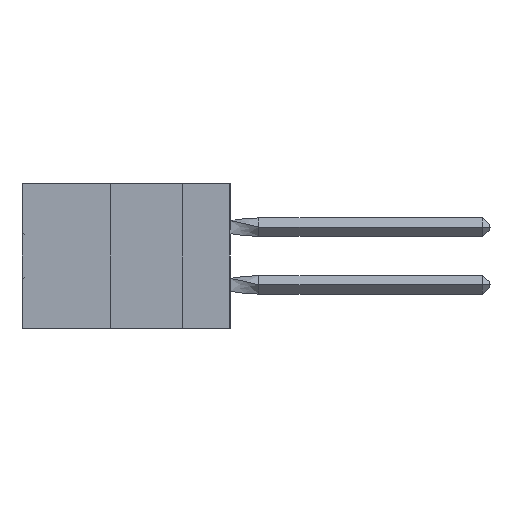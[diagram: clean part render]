
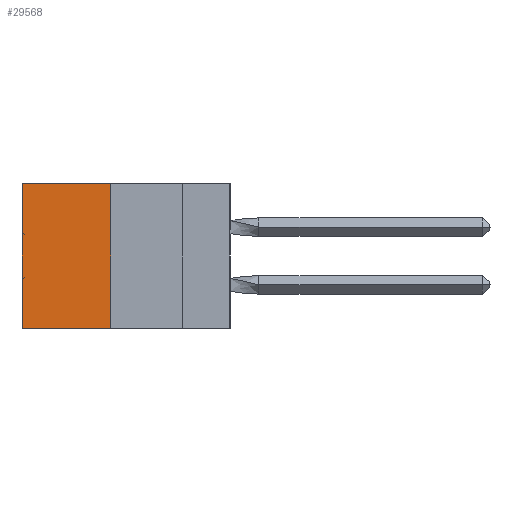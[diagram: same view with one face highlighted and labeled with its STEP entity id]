
A CAD part, left-side view. The second image highlights one B-rep face of the part: STEP entity #29568.
In plain terms, the highlighted planar face has unit normal (-1, 0, 0).
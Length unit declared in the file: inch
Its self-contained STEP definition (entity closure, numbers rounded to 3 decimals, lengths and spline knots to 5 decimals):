
#849 = VECTOR ( 'NONE', #43727, 39.37008 ) ;
#4710 = FACE_OUTER_BOUND ( 'NONE', #11921, .T. ) ;
#4960 = CARTESIAN_POINT ( 'NONE',  ( 0.305, 0.413, -0.5 ) ) ;
#6010 = ORIENTED_EDGE ( 'NONE', *, *, #20643, .F. ) ;
#6087 = EDGE_CURVE ( 'NONE', #27069, #34955, #31797, .T. ) ;
#6821 = EDGE_CURVE ( 'NONE', #34955, #45944, #55097, .T. ) ;
#7483 = ORIENTED_EDGE ( 'NONE', *, *, #6821, .T. ) ;
#8641 = VECTOR ( 'NONE', #21583, 39.37008 ) ;
#11921 = EDGE_LOOP ( 'NONE', ( #7483, #6010, #18293, #22576 ) ) ;
#12285 = PLANE ( 'NONE',  #30268 ) ;
#13831 = CARTESIAN_POINT ( 'NONE',  ( 0.305, 0.72, -0.5 ) ) ;
#15312 = DIRECTION ( 'NONE',  ( 0., 0., -1. ) ) ;
#18049 = CARTESIAN_POINT ( 'NONE',  ( 0.305, 0.72, -0.5 ) ) ;
#18293 = ORIENTED_EDGE ( 'NONE', *, *, #25201, .F. ) ;
#19469 = CARTESIAN_POINT ( 'NONE',  ( 0.305, 0.413, -0.5 ) ) ;
#19927 = CARTESIAN_POINT ( 'NONE',  ( 0.305, 0.72, 0. ) ) ;
#20467 = DIRECTION ( 'NONE',  ( 0., 1., 0. ) ) ;
#20643 = EDGE_CURVE ( 'NONE', #52674, #45944, #23427, .T. ) ;
#21583 = DIRECTION ( 'NONE',  ( 0., 1., 0. ) ) ;
#22576 = ORIENTED_EDGE ( 'NONE', *, *, #6087, .T. ) ;
#23427 = LINE ( 'NONE', #38627, #8641 ) ;
#25201 = EDGE_CURVE ( 'NONE', #27069, #52674, #27667, .T. ) ;
#27069 = VERTEX_POINT ( 'NONE', #51683 ) ;
#27148 = VECTOR ( 'NONE', #20467, 39.37008 ) ;
#27667 = LINE ( 'NONE', #19469, #48987 ) ;
#29043 = DIRECTION ( 'NONE',  ( 1., 0., 0. ) ) ;
#29229 = DIRECTION ( 'NONE',  ( 0., 0., -1. ) ) ;
#29568 = ADVANCED_FACE ( 'NONE', ( #4710 ), #12285, .F. ) ;
#30268 = AXIS2_PLACEMENT_3D ( 'NONE', #46552, #29043, #29229 ) ;
#31797 = LINE ( 'NONE', #46104, #27148 ) ;
#34955 = VERTEX_POINT ( 'NONE', #19927 ) ;
#38627 = CARTESIAN_POINT ( 'NONE',  ( 0.305, 0.413, -0.5 ) ) ;
#43727 = DIRECTION ( 'NONE',  ( 0., 0., -1. ) ) ;
#45944 = VERTEX_POINT ( 'NONE', #13831 ) ;
#46104 = CARTESIAN_POINT ( 'NONE',  ( 0.305, 0.413, 0. ) ) ;
#46552 = CARTESIAN_POINT ( 'NONE',  ( 0.305, 0.413, -0.5 ) ) ;
#48987 = VECTOR ( 'NONE', #15312, 39.37008 ) ;
#51683 = CARTESIAN_POINT ( 'NONE',  ( 0.305, 0.413, 0. ) ) ;
#52674 = VERTEX_POINT ( 'NONE', #4960 ) ;
#55097 = LINE ( 'NONE', #18049, #849 ) ;
